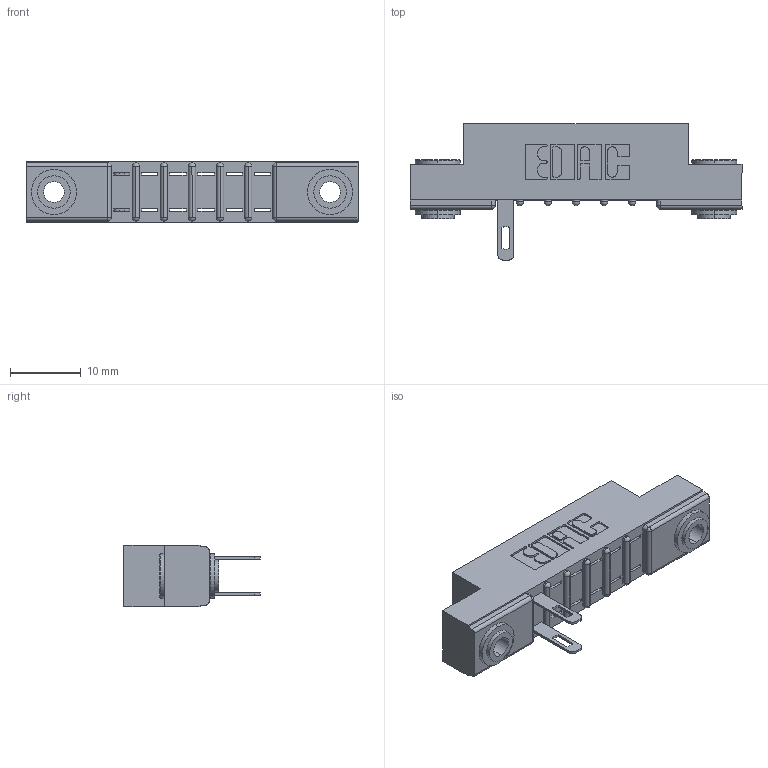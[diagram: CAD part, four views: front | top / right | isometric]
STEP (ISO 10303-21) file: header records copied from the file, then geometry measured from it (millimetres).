
FILE_DESCRIPTION (( 'STEP AP203' ), '1' );
FILE_NAME ('357-012-500-203.STEP', '2018-08-07T21:54:25', ( '' ), ( '' ), 'SwSTEP 2.0', 'SolidWorks 2016', '' );
FILE_SCHEMA (( 'CONFIG_CONTROL_DESIGN' ));
Length unit declared in the file: inch
Products named in the file (4): 345-250-002_345-250-002-102; 357-012-500-203; 307 Part_.156 Dia Mounting Holes; 307-290-001_500
Assembly tree (5 placements, depth 2):
  357-012-500-203
    307 Part_.156 Dia Mounting Holes
    307-290-001_500  x2
    345-250-002_345-250-002-102  x2
Bounding box: 46.79 x 19.18 x 8.71 mm (x, y, z)
Volume: 2939.7 mm3; surface area: 3872.3 mm2
Topology: 5 solids, 5 shells, 369 faces, 1015 edges, 650 vertices
Faces by surface type: plane 214, cylinder 133, sphere 14, cone 8
Entity records: 10493 total; most frequent: CARTESIAN_POINT 1749, DIRECTION 1735, ORIENTED_EDGE 1730, EDGE_CURVE 865, LINE 639, VECTOR 639, VERTEX_POINT 562, AXIS2_PLACEMENT_3D 548
